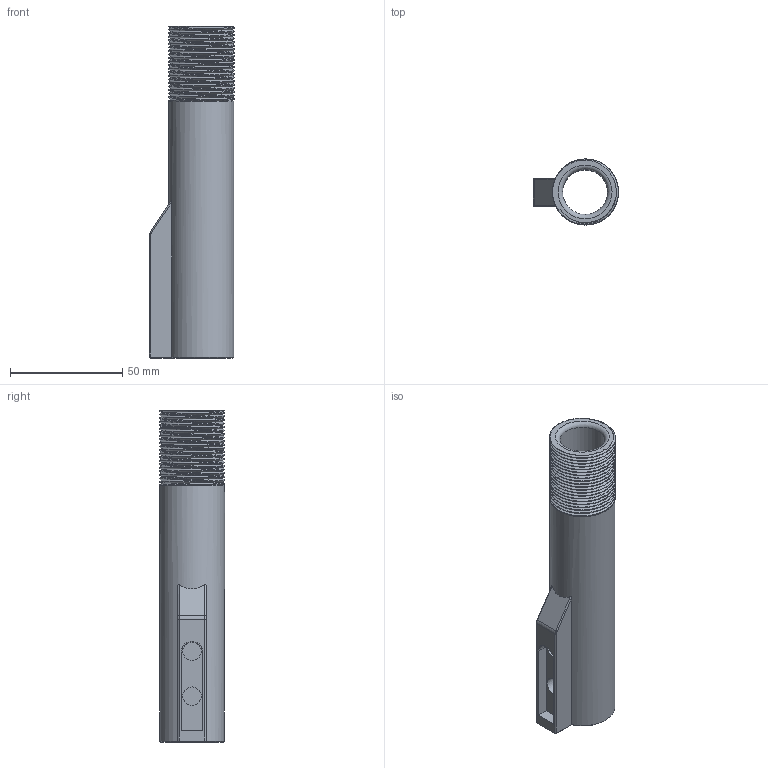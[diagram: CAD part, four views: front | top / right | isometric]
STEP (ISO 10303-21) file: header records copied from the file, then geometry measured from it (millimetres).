
FILE_DESCRIPTION(/* description */ (''),/* implementation_level */ '2;1');
FILE_NAME(/* name */ 'SHORT BUFFER WTF.stp',/* time_stamp */ '2020-05-06T19:02:17+03:00',/* author */ (''),/* organization */ (''),/* preprocessor_version */ 'ST-DEVELOPER v15.2',/* originating_system */ 'Autodesk Translator Framework v2.0.0.5431',/* authorisation */ '');
FILE_SCHEMA (('AUTOMOTIVE_DESIGN { 1 0 10303 214 3 1 1 }'));
Length unit declared in the file: centimetre
Products named in the file (1): SHORT BUFFER
Bounding box: 37.9 x 29.4 x 148 mm (x, y, z)
Volume: 55191.7 mm3; surface area: 27411.1 mm2
Topology: 1 solids, 1 shells, 56 faces, 225 edges, 174 vertices
Faces by surface type: plane 22, bspline 13, cylinder 12, cone 5, torus 4
Full cylindrical faces by diameter (mm): 8.2 x2, 20 x1, 29 x1
Entity records: 13255 total; most frequent: CARTESIAN_POINT 11640, ORIENTED_EDGE 436, EDGE_CURVE 218, DIRECTION 204, VERTEX_POINT 173, B_SPLINE_CURVE_WITH_KNOTS 130, AXIS2_PLACEMENT_3D 83, EDGE_LOOP 67
